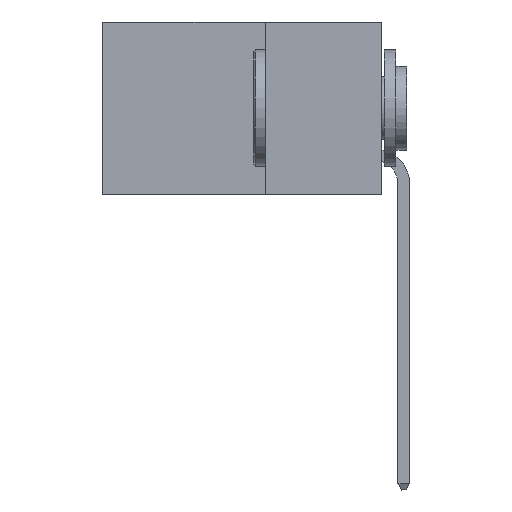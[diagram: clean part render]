
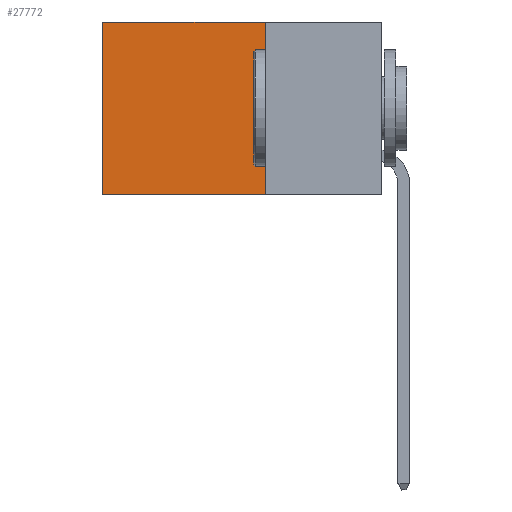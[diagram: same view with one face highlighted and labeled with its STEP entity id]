
A CAD part, left-side view. The second image highlights one B-rep face of the part: STEP entity #27772.
In plain terms, the highlighted planar face has unit normal (-1, 0, 0).
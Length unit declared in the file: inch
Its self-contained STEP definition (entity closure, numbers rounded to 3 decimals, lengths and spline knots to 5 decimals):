
#1125 = ORIENTED_EDGE ( 'NONE', *, *, #23991, .F. ) ;
#2383 = FACE_OUTER_BOUND ( 'NONE', #24687, .T. ) ;
#3042 = CARTESIAN_POINT ( 'NONE',  ( 0.2875, 0.6, 0. ) ) ;
#3995 = EDGE_CURVE ( 'NONE', #8985, #42764, #39643, .T. ) ;
#4124 = CARTESIAN_POINT ( 'NONE',  ( 0.2875, 0.6, 0. ) ) ;
#5026 = VECTOR ( 'NONE', #29643, 39.37008 ) ;
#5035 = PLANE ( 'NONE',  #11404 ) ;
#8629 = DIRECTION ( 'NONE',  ( 1., 0., 0. ) ) ;
#8985 = VERTEX_POINT ( 'NONE', #4124 ) ;
#8994 = ORIENTED_EDGE ( 'NONE', *, *, #31472, .F. ) ;
#10559 = DIRECTION ( 'NONE',  ( 0., 0., -1. ) ) ;
#11404 = AXIS2_PLACEMENT_3D ( 'NONE', #38620, #8629, #27471 ) ;
#12345 = CARTESIAN_POINT ( 'NONE',  ( 0.2875, 0.25, -0.37 ) ) ;
#12829 = CARTESIAN_POINT ( 'NONE',  ( 0.2875, 0.6, -0.37 ) ) ;
#14978 = EDGE_CURVE ( 'NONE', #34420, #8985, #30823, .T. ) ;
#18118 = CARTESIAN_POINT ( 'NONE',  ( 0.2875, 0.25, -0.37 ) ) ;
#19870 = DIRECTION ( 'NONE',  ( 0., 1., 0. ) ) ;
#22371 = VECTOR ( 'NONE', #36802, 39.37008 ) ;
#23991 = EDGE_CURVE ( 'NONE', #45924, #42764, #36458, .T. ) ;
#24193 = CARTESIAN_POINT ( 'NONE',  ( 0.2875, 0.25, 0. ) ) ;
#24687 = EDGE_LOOP ( 'NONE', ( #27592, #1125, #8994, #45482 ) ) ;
#27294 = VECTOR ( 'NONE', #19870, 39.37008 ) ;
#27471 = DIRECTION ( 'NONE',  ( 0., 0., -1. ) ) ;
#27592 = ORIENTED_EDGE ( 'NONE', *, *, #3995, .T. ) ;
#27772 = ADVANCED_FACE ( 'NONE', ( #2383 ), #5035, .F. ) ;
#29643 = DIRECTION ( 'NONE',  ( 0., 0., -1. ) ) ;
#30204 = LINE ( 'NONE', #40155, #5026 ) ;
#30823 = LINE ( 'NONE', #47266, #27294 ) ;
#31472 = EDGE_CURVE ( 'NONE', #34420, #45924, #30204, .T. ) ;
#34420 = VERTEX_POINT ( 'NONE', #24193 ) ;
#36458 = LINE ( 'NONE', #18118, #22371 ) ;
#36802 = DIRECTION ( 'NONE',  ( 0., 1., 0. ) ) ;
#38620 = CARTESIAN_POINT ( 'NONE',  ( 0.2875, 0.25, 0. ) ) ;
#39643 = LINE ( 'NONE', #3042, #46725 ) ;
#40155 = CARTESIAN_POINT ( 'NONE',  ( 0.2875, 0.25, 0. ) ) ;
#42764 = VERTEX_POINT ( 'NONE', #12829 ) ;
#45482 = ORIENTED_EDGE ( 'NONE', *, *, #14978, .T. ) ;
#45924 = VERTEX_POINT ( 'NONE', #12345 ) ;
#46725 = VECTOR ( 'NONE', #10559, 39.37008 ) ;
#47266 = CARTESIAN_POINT ( 'NONE',  ( 0.2875, 0.25, 0. ) ) ;
